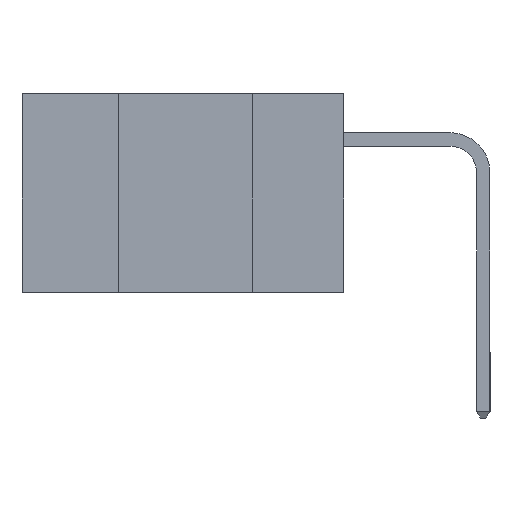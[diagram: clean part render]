
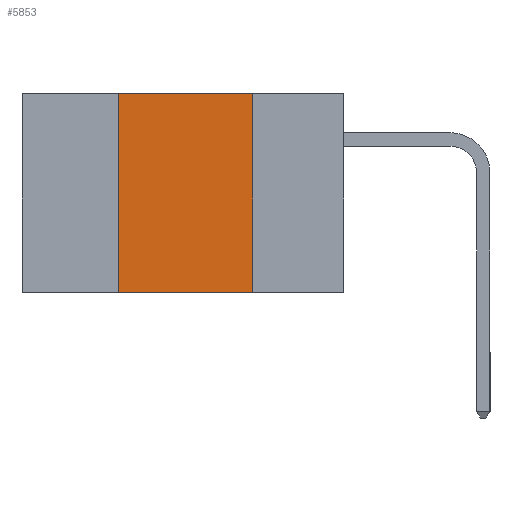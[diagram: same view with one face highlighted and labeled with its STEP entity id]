
A CAD part, left-side view. The second image highlights one B-rep face of the part: STEP entity #5853.
In plain terms, the highlighted planar face has unit normal (-1, 0, 0).
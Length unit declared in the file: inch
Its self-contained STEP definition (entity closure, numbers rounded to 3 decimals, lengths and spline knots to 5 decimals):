
#620 = EDGE_CURVE ( 'NONE', #9087, #9684, #2650, .T. ) ;
#885 = ORIENTED_EDGE ( 'NONE', *, *, #4823, .T. ) ;
#952 = ORIENTED_EDGE ( 'NONE', *, *, #6954, .F. ) ;
#1262 = EDGE_LOOP ( 'NONE', ( #2835, #952, #1754, #885 ) ) ;
#1754 = ORIENTED_EDGE ( 'NONE', *, *, #620, .F. ) ;
#1879 = CARTESIAN_POINT ( 'NONE',  ( 0., 0.42, 0. ) ) ;
#2650 = LINE ( 'NONE', #9495, #3273 ) ;
#2835 = ORIENTED_EDGE ( 'NONE', *, *, #8866, .F. ) ;
#3273 = VECTOR ( 'NONE', #5314, 39.37008 ) ;
#3944 = LINE ( 'NONE', #10658, #6905 ) ;
#4823 = EDGE_CURVE ( 'NONE', #9087, #10569, #9997, .T. ) ;
#5314 = DIRECTION ( 'NONE',  ( 0., 0., 1. ) ) ;
#5806 = LINE ( 'NONE', #9977, #7745 ) ;
#5853 = ADVANCED_FACE ( 'NONE', ( #9453 ), #6274, .F. ) ;
#5876 = DIRECTION ( 'NONE',  ( 0., -1., 0. ) ) ;
#6138 = AXIS2_PLACEMENT_3D ( 'NONE', #8640, #7160, #9616 ) ;
#6274 = PLANE ( 'NONE',  #6138 ) ;
#6487 = DIRECTION ( 'NONE',  ( 0., 0., -1. ) ) ;
#6698 = CARTESIAN_POINT ( 'NONE',  ( 0., 0.17, -0.37 ) ) ;
#6725 = DIRECTION ( 'NONE',  ( 0., -1., 0. ) ) ;
#6905 = VECTOR ( 'NONE', #6487, 39.37008 ) ;
#6954 = EDGE_CURVE ( 'NONE', #9684, #8982, #5806, .T. ) ;
#7160 = DIRECTION ( 'NONE',  ( 1., 0., 0. ) ) ;
#7621 = CARTESIAN_POINT ( 'NONE',  ( 0., 0.6, -0.37 ) ) ;
#7745 = VECTOR ( 'NONE', #6725, 39.37008 ) ;
#7823 = CARTESIAN_POINT ( 'NONE',  ( 0., 0.42, -0.37 ) ) ;
#8640 = CARTESIAN_POINT ( 'NONE',  ( 0., 0.6, 0. ) ) ;
#8866 = EDGE_CURVE ( 'NONE', #8982, #10569, #3944, .T. ) ;
#8982 = VERTEX_POINT ( 'NONE', #10888 ) ;
#9087 = VERTEX_POINT ( 'NONE', #7823 ) ;
#9453 = FACE_OUTER_BOUND ( 'NONE', #1262, .T. ) ;
#9495 = CARTESIAN_POINT ( 'NONE',  ( 0., 0.42, -0.37 ) ) ;
#9616 = DIRECTION ( 'NONE',  ( 0., 0., -1. ) ) ;
#9684 = VERTEX_POINT ( 'NONE', #1879 ) ;
#9977 = CARTESIAN_POINT ( 'NONE',  ( 0., 0.6, 0. ) ) ;
#9997 = LINE ( 'NONE', #7621, #10316 ) ;
#10316 = VECTOR ( 'NONE', #5876, 39.37008 ) ;
#10569 = VERTEX_POINT ( 'NONE', #6698 ) ;
#10658 = CARTESIAN_POINT ( 'NONE',  ( 0., 0.17, -0.37 ) ) ;
#10888 = CARTESIAN_POINT ( 'NONE',  ( 0., 0.17, 0. ) ) ;
